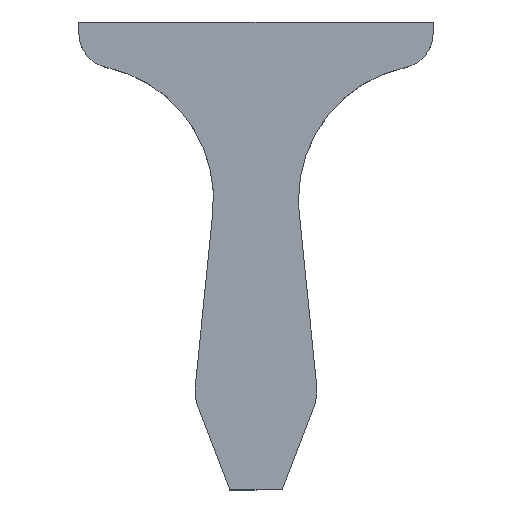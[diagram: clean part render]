
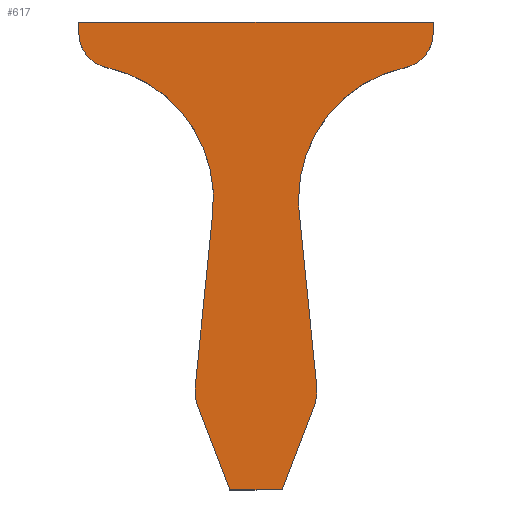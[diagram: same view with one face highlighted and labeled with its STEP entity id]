
A CAD part, top view. The second image highlights one B-rep face of the part: STEP entity #617.
In plain terms, the highlighted planar face has unit normal (0, 0, 1).
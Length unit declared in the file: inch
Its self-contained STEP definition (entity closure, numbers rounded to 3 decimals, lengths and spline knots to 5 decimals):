
#5 = CARTESIAN_POINT ( 'NONE',  ( -0.04097, -0.01104, 0.045 ) ) ;
#13 = CARTESIAN_POINT ( 'NONE',  ( -0.125, 0.135, 0.045 ) ) ;
#15 = LINE ( 'NONE', #447, #609 ) ;
#22 = VERTEX_POINT ( 'NONE', #446 ) ;
#23 = LINE ( 'NONE', #103, #181 ) ;
#35 = DIRECTION ( 'NONE',  ( 0., 0., -1. ) ) ;
#42 = EDGE_CURVE ( 'NONE', #394, #125, #380, .T. ) ;
#45 = VECTOR ( 'NONE', #202, 39.37008 ) ;
#55 = EDGE_CURVE ( 'NONE', #578, #404, #411, .T. ) ;
#59 = EDGE_CURVE ( 'NONE', #507, #277, #187, .T. ) ;
#60 = CARTESIAN_POINT ( 'NONE',  ( -0.012, 0., 0.045 ) ) ;
#65 = DIRECTION ( 'NONE',  ( 0.356, 0.934, 0. ) ) ;
#69 = CARTESIAN_POINT ( 'NONE',  ( 0.125, 0.135, 0.045 ) ) ;
#72 = VERTEX_POINT ( 'NONE', #407 ) ;
#74 = VERTEX_POINT ( 'NONE', #363 ) ;
#75 = DIRECTION ( 'NONE',  ( -0.101, 0.995, 0. ) ) ;
#77 = ORIENTED_EDGE ( 'NONE', *, *, #437, .T. ) ;
#84 = DIRECTION ( 'NONE',  ( 0., -1., 0. ) ) ;
#88 = AXIS2_PLACEMENT_3D ( 'NONE', #13, #35, #226 ) ;
#90 = VECTOR ( 'NONE', #223, 39.37008 ) ;
#98 = LINE ( 'NONE', #5, #481 ) ;
#103 = CARTESIAN_POINT ( 'NONE',  ( 0.04097, -0.01104, 0.045 ) ) ;
#106 = ORIENTED_EDGE ( 'NONE', *, *, #422, .T. ) ;
#110 = DIRECTION ( 'NONE',  ( 0., 0., 1. ) ) ;
#111 = ORIENTED_EDGE ( 'NONE', *, *, #395, .T. ) ;
#118 = DIRECTION ( 'NONE',  ( -1., 0., 0. ) ) ;
#125 = VERTEX_POINT ( 'NONE', #133 ) ;
#129 = AXIS2_PLACEMENT_3D ( 'NONE', #60, #110, #409 ) ;
#132 = CARTESIAN_POINT ( 'NONE',  ( -0.125, 0.26, 0.045 ) ) ;
#133 = CARTESIAN_POINT ( 'NONE',  ( -0.03048, 0.12545, 0.045 ) ) ;
#136 = DIRECTION ( 'NONE',  ( 1., 0., 0. ) ) ;
#139 = CARTESIAN_POINT ( 'NONE',  ( 0.1, 0.25237, 0.045 ) ) ;
#141 = AXIS2_PLACEMENT_3D ( 'NONE', #303, #317, #442 ) ;
#152 = DIRECTION ( 'NONE',  ( 0., 0., -1. ) ) ;
#157 = ORIENTED_EDGE ( 'NONE', *, *, #192, .T. ) ;
#162 = ORIENTED_EDGE ( 'NONE', *, *, #59, .T. ) ;
#167 = EDGE_LOOP ( 'NONE', ( #77, #453, #460, #516, #191, #111, #157, #546, #219, #162, #275, #621, #552, #513, #243, #106 ) ) ;
#175 = CARTESIAN_POINT ( 'NONE',  ( 0.125, 0.135, 0.045 ) ) ;
#181 = VECTOR ( 'NONE', #65, 39.37008 ) ;
#183 = DIRECTION ( 'NONE',  ( 0., 0., -1. ) ) ;
#186 = CARTESIAN_POINT ( 'NONE',  ( 0.03, 0.135, 0.045 ) ) ;
#187 = CIRCLE ( 'NONE', #298, 0.031 ) ;
#191 = ORIENTED_EDGE ( 'NONE', *, *, #391, .T. ) ;
#192 = EDGE_CURVE ( 'NONE', #443, #591, #98, .T. ) ;
#194 = AXIS2_PLACEMENT_3D ( 'NONE', #343, #338, #619 ) ;
#195 = AXIS2_PLACEMENT_3D ( 'NONE', #199, #537, #250 ) ;
#199 = CARTESIAN_POINT ( 'NONE',  ( -0.1, 0.25237, 0.045 ) ) ;
#202 = DIRECTION ( 'NONE',  ( 1., 0., 0. ) ) ;
#204 = VECTOR ( 'NONE', #118, 39.37008 ) ;
#213 = VERTEX_POINT ( 'NONE', #587 ) ;
#218 = CARTESIAN_POINT ( 'NONE',  ( 0.0185, -0.07, 0.045 ) ) ;
#219 = ORIENTED_EDGE ( 'NONE', *, *, #376, .T. ) ;
#223 = DIRECTION ( 'NONE',  ( 0., 1., 0. ) ) ;
#226 = DIRECTION ( 'NONE',  ( -1., 0., 0. ) ) ;
#234 = VECTOR ( 'NONE', #84, 39.37008 ) ;
#239 = CARTESIAN_POINT ( 'NONE',  ( -0.04097, -0.01104, 0.045 ) ) ;
#243 = ORIENTED_EDGE ( 'NONE', *, *, #293, .T. ) ;
#244 = EDGE_CURVE ( 'NONE', #591, #322, #344, .T. ) ;
#250 = DIRECTION ( 'NONE',  ( 1., 0., 0. ) ) ;
#255 = DIRECTION ( 'NONE',  ( 0.356, -0.934, 0. ) ) ;
#257 = LINE ( 'NONE', #602, #204 ) ;
#266 = CARTESIAN_POINT ( 'NONE',  ( 0.04284, 0.00312, 0.045 ) ) ;
#275 = ORIENTED_EDGE ( 'NONE', *, *, #301, .T. ) ;
#277 = VERTEX_POINT ( 'NONE', #266 ) ;
#278 = EDGE_CURVE ( 'NONE', #318, #394, #415, .T. ) ;
#287 = AXIS2_PLACEMENT_3D ( 'NONE', #139, #430, #580 ) ;
#293 = EDGE_CURVE ( 'NONE', #297, #74, #585, .T. ) ;
#297 = VERTEX_POINT ( 'NONE', #558 ) ;
#298 = AXIS2_PLACEMENT_3D ( 'NONE', #352, #544, #457 ) ;
#301 = EDGE_CURVE ( 'NONE', #277, #22, #15, .T. ) ;
#303 = CARTESIAN_POINT ( 'NONE',  ( -0.012, 0., 0.045 ) ) ;
#312 = CIRCLE ( 'NONE', #334, 0.095 ) ;
#317 = DIRECTION ( 'NONE',  ( 0., 0., 1. ) ) ;
#318 = VERTEX_POINT ( 'NONE', #454 ) ;
#321 = DIRECTION ( 'NONE',  ( -0.101, -0.995, 0. ) ) ;
#322 = VERTEX_POINT ( 'NONE', #218 ) ;
#324 = CARTESIAN_POINT ( 'NONE',  ( -0.125, 0.26, 0.045 ) ) ;
#334 = AXIS2_PLACEMENT_3D ( 'NONE', #175, #183, #136 ) ;
#338 = DIRECTION ( 'NONE',  ( 0., 0., 1. ) ) ;
#343 = CARTESIAN_POINT ( 'NONE',  ( -0.1, 0.25237, 0.045 ) ) ;
#344 = LINE ( 'NONE', #500, #45 ) ;
#352 = CARTESIAN_POINT ( 'NONE',  ( 0.012, 0., 0.045 ) ) ;
#353 = LINE ( 'NONE', #545, #615 ) ;
#363 = CARTESIAN_POINT ( 'NONE',  ( 0.125, 0.26, 0.045 ) ) ;
#372 = LINE ( 'NONE', #132, #234 ) ;
#374 = CARTESIAN_POINT ( 'NONE',  ( 0.04097, -0.01104, 0.045 ) ) ;
#376 = EDGE_CURVE ( 'NONE', #322, #507, #23, .T. ) ;
#380 = CIRCLE ( 'NONE', #88, 0.095 ) ;
#382 = EDGE_CURVE ( 'NONE', #125, #72, #353, .T. ) ;
#383 = FACE_OUTER_BOUND ( 'NONE', #167, .T. ) ;
#391 = EDGE_CURVE ( 'NONE', #72, #213, #501, .T. ) ;
#394 = VERTEX_POINT ( 'NONE', #493 ) ;
#395 = EDGE_CURVE ( 'NONE', #213, #443, #479, .T. ) ;
#404 = VERTEX_POINT ( 'NONE', #506 ) ;
#407 = CARTESIAN_POINT ( 'NONE',  ( -0.04284, 0.00312, 0.045 ) ) ;
#409 = DIRECTION ( 'NONE',  ( 1., 0., 0. ) ) ;
#411 = CIRCLE ( 'NONE', #465, 0.095 ) ;
#412 = CIRCLE ( 'NONE', #287, 0.025 ) ;
#415 = CIRCLE ( 'NONE', #195, 0.025 ) ;
#422 = EDGE_CURVE ( 'NONE', #74, #494, #257, .T. ) ;
#430 = DIRECTION ( 'NONE',  ( 0., 0., 1. ) ) ;
#437 = EDGE_CURVE ( 'NONE', #494, #318, #372, .T. ) ;
#442 = DIRECTION ( 'NONE',  ( 1., 0., 0. ) ) ;
#443 = VERTEX_POINT ( 'NONE', #239 ) ;
#446 = CARTESIAN_POINT ( 'NONE',  ( 0.03048, 0.12545, 0.045 ) ) ;
#447 = CARTESIAN_POINT ( 'NONE',  ( 0.03048, 0.12545, 0.045 ) ) ;
#453 = ORIENTED_EDGE ( 'NONE', *, *, #278, .T. ) ;
#454 = CARTESIAN_POINT ( 'NONE',  ( -0.125, 0.25237, 0.045 ) ) ;
#457 = DIRECTION ( 'NONE',  ( -1., 0., 0. ) ) ;
#460 = ORIENTED_EDGE ( 'NONE', *, *, #42, .T. ) ;
#465 = AXIS2_PLACEMENT_3D ( 'NONE', #69, #152, #549 ) ;
#479 = CIRCLE ( 'NONE', #129, 0.031 ) ;
#481 = VECTOR ( 'NONE', #255, 39.37008 ) ;
#493 = CARTESIAN_POINT ( 'NONE',  ( -0.10521, 0.22792, 0.045 ) ) ;
#494 = VERTEX_POINT ( 'NONE', #324 ) ;
#500 = CARTESIAN_POINT ( 'NONE',  ( -0.0185, -0.07, 0.045 ) ) ;
#501 = CIRCLE ( 'NONE', #141, 0.031 ) ;
#506 = CARTESIAN_POINT ( 'NONE',  ( 0.10521, 0.22792, 0.045 ) ) ;
#507 = VERTEX_POINT ( 'NONE', #374 ) ;
#513 = ORIENTED_EDGE ( 'NONE', *, *, #594, .T. ) ;
#516 = ORIENTED_EDGE ( 'NONE', *, *, #382, .T. ) ;
#519 = EDGE_CURVE ( 'NONE', #22, #578, #312, .T. ) ;
#537 = DIRECTION ( 'NONE',  ( 0., 0., 1. ) ) ;
#544 = DIRECTION ( 'NONE',  ( 0., 0., 1. ) ) ;
#545 = CARTESIAN_POINT ( 'NONE',  ( -0.03048, 0.12545, 0.045 ) ) ;
#546 = ORIENTED_EDGE ( 'NONE', *, *, #244, .T. ) ;
#549 = DIRECTION ( 'NONE',  ( 1., 0., 0. ) ) ;
#551 = CARTESIAN_POINT ( 'NONE',  ( 0.125, 0.26, 0.045 ) ) ;
#552 = ORIENTED_EDGE ( 'NONE', *, *, #55, .T. ) ;
#558 = CARTESIAN_POINT ( 'NONE',  ( 0.125, 0.25237, 0.045 ) ) ;
#578 = VERTEX_POINT ( 'NONE', #186 ) ;
#580 = DIRECTION ( 'NONE',  ( -1., 0., 0. ) ) ;
#585 = LINE ( 'NONE', #551, #90 ) ;
#587 = CARTESIAN_POINT ( 'NONE',  ( -0.043, 0., 0.045 ) ) ;
#591 = VERTEX_POINT ( 'NONE', #623 ) ;
#594 = EDGE_CURVE ( 'NONE', #404, #297, #412, .T. ) ;
#602 = CARTESIAN_POINT ( 'NONE',  ( -0.125, 0.26, 0.045 ) ) ;
#609 = VECTOR ( 'NONE', #75, 39.37008 ) ;
#615 = VECTOR ( 'NONE', #321, 39.37008 ) ;
#617 = ADVANCED_FACE ( 'NONE', ( #383 ), #620, .T. ) ;
#619 = DIRECTION ( 'NONE',  ( 1., 0., 0. ) ) ;
#620 = PLANE ( 'NONE',  #194 ) ;
#621 = ORIENTED_EDGE ( 'NONE', *, *, #519, .T. ) ;
#623 = CARTESIAN_POINT ( 'NONE',  ( -0.0185, -0.07, 0.045 ) ) ;
